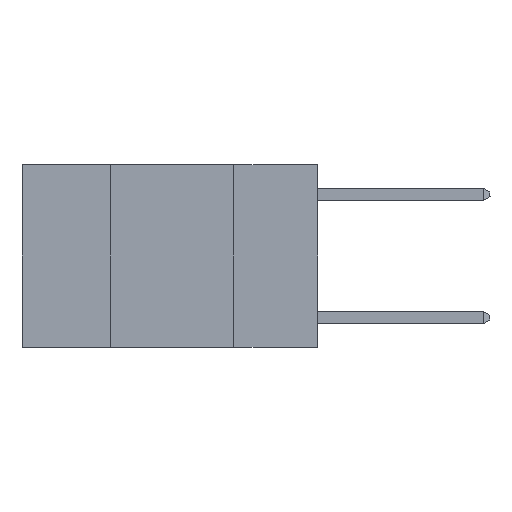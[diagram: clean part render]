
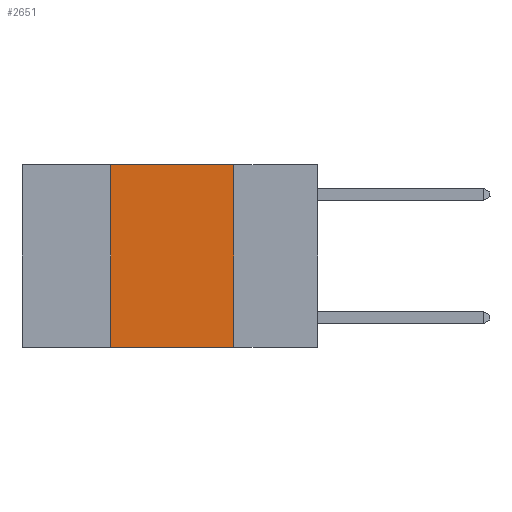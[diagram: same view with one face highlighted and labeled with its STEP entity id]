
A CAD part, left-side view. The second image highlights one B-rep face of the part: STEP entity #2651.
In plain terms, the highlighted planar face has unit normal (-1, 0, 0).
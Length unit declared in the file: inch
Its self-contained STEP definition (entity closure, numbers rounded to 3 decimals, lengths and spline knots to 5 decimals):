
#41 = VECTOR ( 'NONE', #6392, 39.37008 ) ;
#396 = AXIS2_PLACEMENT_3D ( 'NONE', #9639, #11630, #8664 ) ;
#978 = EDGE_CURVE ( 'NONE', #5802, #10525, #13146, .T. ) ;
#1379 = ORIENTED_EDGE ( 'NONE', *, *, #10341, .F. ) ;
#1508 = ORIENTED_EDGE ( 'NONE', *, *, #978, .T. ) ;
#2156 = PLANE ( 'NONE',  #396 ) ;
#2233 = VECTOR ( 'NONE', #12100, 39.37008 ) ;
#2385 = LINE ( 'NONE', #10811, #11837 ) ;
#2651 = ADVANCED_FACE ( 'NONE', ( #9705 ), #2156, .F. ) ;
#2825 = DIRECTION ( 'NONE',  ( 0., -1., 0. ) ) ;
#3506 = CARTESIAN_POINT ( 'NONE',  ( 0., 0.42, 0. ) ) ;
#3507 = EDGE_CURVE ( 'NONE', #4672, #10525, #2385, .T. ) ;
#3579 = VERTEX_POINT ( 'NONE', #3506 ) ;
#3872 = CARTESIAN_POINT ( 'NONE',  ( 0., 0.6, -0.37 ) ) ;
#4462 = EDGE_CURVE ( 'NONE', #3579, #4672, #11089, .T. ) ;
#4672 = VERTEX_POINT ( 'NONE', #9931 ) ;
#5001 = CARTESIAN_POINT ( 'NONE',  ( 0., 0.6, 0. ) ) ;
#5802 = VERTEX_POINT ( 'NONE', #13147 ) ;
#6392 = DIRECTION ( 'NONE',  ( 0., 0., 1. ) ) ;
#8222 = ORIENTED_EDGE ( 'NONE', *, *, #3507, .F. ) ;
#8649 = LINE ( 'NONE', #12532, #41 ) ;
#8664 = DIRECTION ( 'NONE',  ( 0., 0., -1. ) ) ;
#9216 = ORIENTED_EDGE ( 'NONE', *, *, #4462, .F. ) ;
#9394 = EDGE_LOOP ( 'NONE', ( #8222, #9216, #1379, #1508 ) ) ;
#9639 = CARTESIAN_POINT ( 'NONE',  ( 0., 0.6, 0. ) ) ;
#9705 = FACE_OUTER_BOUND ( 'NONE', #9394, .T. ) ;
#9931 = CARTESIAN_POINT ( 'NONE',  ( 0., 0.17, 0. ) ) ;
#10341 = EDGE_CURVE ( 'NONE', #5802, #3579, #8649, .T. ) ;
#10525 = VERTEX_POINT ( 'NONE', #12986 ) ;
#10811 = CARTESIAN_POINT ( 'NONE',  ( 0., 0.17, 0. ) ) ;
#10907 = VECTOR ( 'NONE', #2825, 39.37008 ) ;
#11089 = LINE ( 'NONE', #5001, #2233 ) ;
#11630 = DIRECTION ( 'NONE',  ( 1., 0., 0. ) ) ;
#11837 = VECTOR ( 'NONE', #12712, 39.37008 ) ;
#12100 = DIRECTION ( 'NONE',  ( 0., -1., 0. ) ) ;
#12532 = CARTESIAN_POINT ( 'NONE',  ( 0., 0.42, 0. ) ) ;
#12712 = DIRECTION ( 'NONE',  ( 0., 0., -1. ) ) ;
#12986 = CARTESIAN_POINT ( 'NONE',  ( 0., 0.17, -0.37 ) ) ;
#13146 = LINE ( 'NONE', #3872, #10907 ) ;
#13147 = CARTESIAN_POINT ( 'NONE',  ( 0., 0.42, -0.37 ) ) ;
